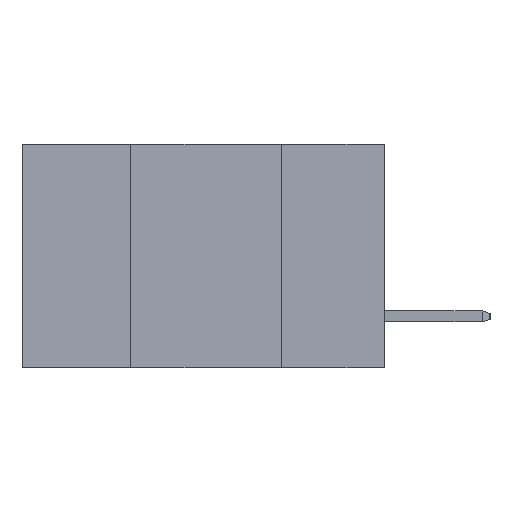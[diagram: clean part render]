
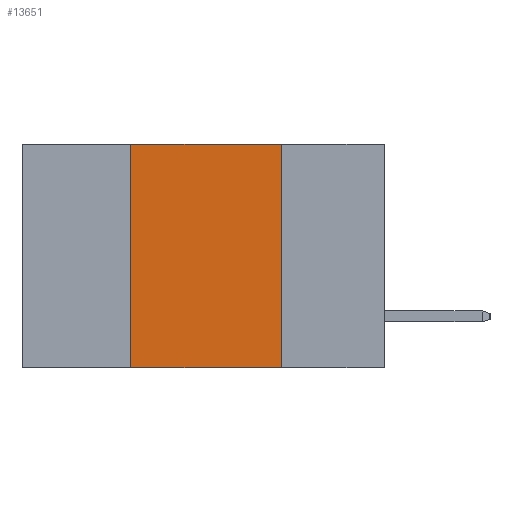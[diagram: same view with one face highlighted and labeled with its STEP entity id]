
A CAD part, left-side view. The second image highlights one B-rep face of the part: STEP entity #13651.
In plain terms, the highlighted planar face has unit normal (-1, 0, 0).
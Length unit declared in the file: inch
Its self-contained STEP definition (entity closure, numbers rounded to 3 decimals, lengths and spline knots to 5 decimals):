
#458 = VECTOR ( 'NONE', #18977, 39.37008 ) ;
#970 = VECTOR ( 'NONE', #2734, 39.37008 ) ;
#1570 = ORIENTED_EDGE ( 'NONE', *, *, #21559, .F. ) ;
#2734 = DIRECTION ( 'NONE',  ( 0., 0., 1. ) ) ;
#3217 = CARTESIAN_POINT ( 'NONE',  ( 0., 0.42, -0.37 ) ) ;
#5004 = EDGE_CURVE ( 'NONE', #7426, #11449, #19093, .T. ) ;
#5043 = ORIENTED_EDGE ( 'NONE', *, *, #5004, .F. ) ;
#5107 = FACE_OUTER_BOUND ( 'NONE', #15038, .T. ) ;
#5718 = EDGE_CURVE ( 'NONE', #12809, #7426, #9013, .T. ) ;
#6030 = LINE ( 'NONE', #3217, #970 ) ;
#6327 = DIRECTION ( 'NONE',  ( 0., -1., 0. ) ) ;
#7426 = VERTEX_POINT ( 'NONE', #19353 ) ;
#9013 = LINE ( 'NONE', #19783, #458 ) ;
#9029 = VERTEX_POINT ( 'NONE', #20590 ) ;
#10704 = CARTESIAN_POINT ( 'NONE',  ( 0., 0.6, 0. ) ) ;
#10709 = CARTESIAN_POINT ( 'NONE',  ( 0., 0.6, -0.37 ) ) ;
#10735 = DIRECTION ( 'NONE',  ( 0., 0., -1. ) ) ;
#10792 = DIRECTION ( 'NONE',  ( 1., 0., 0. ) ) ;
#10814 = PLANE ( 'NONE',  #19187 ) ;
#11449 = VERTEX_POINT ( 'NONE', #19007 ) ;
#12331 = VECTOR ( 'NONE', #6327, 39.37008 ) ;
#12495 = EDGE_CURVE ( 'NONE', #9029, #11449, #17192, .T. ) ;
#12809 = VERTEX_POINT ( 'NONE', #21232 ) ;
#13651 = ADVANCED_FACE ( 'NONE', ( #5107 ), #10814, .F. ) ;
#13997 = ORIENTED_EDGE ( 'NONE', *, *, #12495, .T. ) ;
#14760 = VECTOR ( 'NONE', #16570, 39.37008 ) ;
#15038 = EDGE_LOOP ( 'NONE', ( #5043, #17286, #1570, #13997 ) ) ;
#16168 = CARTESIAN_POINT ( 'NONE',  ( 0., 0.17, -0.37 ) ) ;
#16570 = DIRECTION ( 'NONE',  ( 0., 0., -1. ) ) ;
#17192 = LINE ( 'NONE', #10709, #12331 ) ;
#17286 = ORIENTED_EDGE ( 'NONE', *, *, #5718, .F. ) ;
#18977 = DIRECTION ( 'NONE',  ( 0., -1., 0. ) ) ;
#19007 = CARTESIAN_POINT ( 'NONE',  ( 0., 0.17, -0.37 ) ) ;
#19093 = LINE ( 'NONE', #16168, #14760 ) ;
#19187 = AXIS2_PLACEMENT_3D ( 'NONE', #10704, #10792, #10735 ) ;
#19353 = CARTESIAN_POINT ( 'NONE',  ( 0., 0.17, 0. ) ) ;
#19783 = CARTESIAN_POINT ( 'NONE',  ( 0., 0.6, 0. ) ) ;
#20590 = CARTESIAN_POINT ( 'NONE',  ( 0., 0.42, -0.37 ) ) ;
#21232 = CARTESIAN_POINT ( 'NONE',  ( 0., 0.42, 0. ) ) ;
#21559 = EDGE_CURVE ( 'NONE', #9029, #12809, #6030, .T. ) ;
